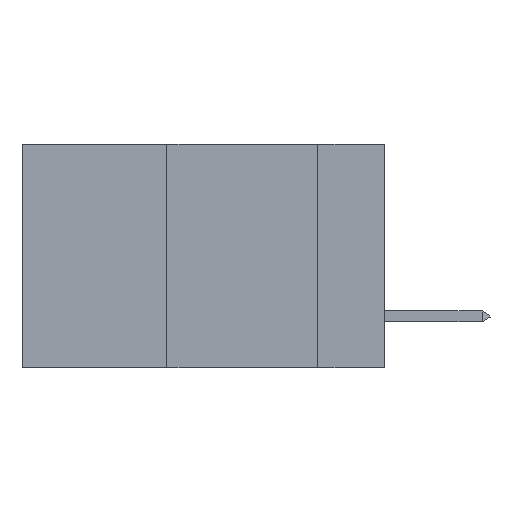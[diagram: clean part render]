
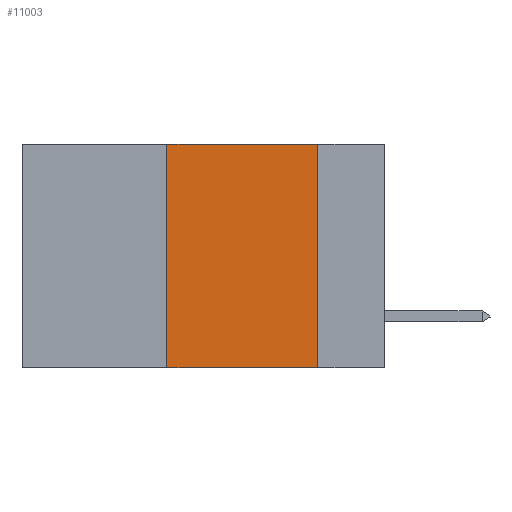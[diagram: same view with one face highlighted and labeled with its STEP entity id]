
A CAD part, left-side view. The second image highlights one B-rep face of the part: STEP entity #11003.
In plain terms, the highlighted planar face has unit normal (-1, 0, 0).
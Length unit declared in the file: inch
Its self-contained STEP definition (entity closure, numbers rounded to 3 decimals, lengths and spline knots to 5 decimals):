
#682 = VECTOR ( 'NONE', #30937, 39.37008 ) ;
#923 = PLANE ( 'NONE',  #15799 ) ;
#1161 = FACE_OUTER_BOUND ( 'NONE', #6146, .T. ) ;
#1852 = LINE ( 'NONE', #16204, #682 ) ;
#6146 = EDGE_LOOP ( 'NONE', ( #11943, #43986, #10461, #16983 ) ) ;
#6515 = LINE ( 'NONE', #18355, #30568 ) ;
#7495 = VECTOR ( 'NONE', #24805, 39.37008 ) ;
#9972 = EDGE_CURVE ( 'NONE', #40514, #22661, #1852, .T. ) ;
#10461 = ORIENTED_EDGE ( 'NONE', *, *, #11871, .F. ) ;
#11003 = ADVANCED_FACE ( 'NONE', ( #1161 ), #923, .F. ) ;
#11871 = EDGE_CURVE ( 'NONE', #40514, #37685, #32154, .T. ) ;
#11943 = ORIENTED_EDGE ( 'NONE', *, *, #27723, .F. ) ;
#12066 = DIRECTION ( 'NONE',  ( 0., 0., -1. ) ) ;
#14616 = CARTESIAN_POINT ( 'NONE',  ( 0., 0.6, 0. ) ) ;
#15799 = AXIS2_PLACEMENT_3D ( 'NONE', #30419, #22915, #12066 ) ;
#16204 = CARTESIAN_POINT ( 'NONE',  ( 0., 0.6, -0.37 ) ) ;
#16643 = CARTESIAN_POINT ( 'NONE',  ( 0., 0.36, 0. ) ) ;
#16983 = ORIENTED_EDGE ( 'NONE', *, *, #9972, .T. ) ;
#18355 = CARTESIAN_POINT ( 'NONE',  ( 0., 0.11, 0. ) ) ;
#22661 = VERTEX_POINT ( 'NONE', #30982 ) ;
#22915 = DIRECTION ( 'NONE',  ( 1., 0., 0. ) ) ;
#24805 = DIRECTION ( 'NONE',  ( 0., 0., 1. ) ) ;
#25208 = VECTOR ( 'NONE', #37719, 39.37008 ) ;
#25822 = VERTEX_POINT ( 'NONE', #32988 ) ;
#27723 = EDGE_CURVE ( 'NONE', #25822, #22661, #6515, .T. ) ;
#29859 = CARTESIAN_POINT ( 'NONE',  ( 0., 0.36, 0. ) ) ;
#30419 = CARTESIAN_POINT ( 'NONE',  ( 0., 0.6, 0. ) ) ;
#30420 = CARTESIAN_POINT ( 'NONE',  ( 0., 0.36, -0.37 ) ) ;
#30568 = VECTOR ( 'NONE', #33601, 39.37008 ) ;
#30937 = DIRECTION ( 'NONE',  ( 0., -1., 0. ) ) ;
#30982 = CARTESIAN_POINT ( 'NONE',  ( 0., 0.11, -0.37 ) ) ;
#32154 = LINE ( 'NONE', #29859, #7495 ) ;
#32988 = CARTESIAN_POINT ( 'NONE',  ( 0., 0.11, 0. ) ) ;
#33601 = DIRECTION ( 'NONE',  ( 0., 0., -1. ) ) ;
#37685 = VERTEX_POINT ( 'NONE', #16643 ) ;
#37719 = DIRECTION ( 'NONE',  ( 0., -1., 0. ) ) ;
#38711 = LINE ( 'NONE', #14616, #25208 ) ;
#40514 = VERTEX_POINT ( 'NONE', #30420 ) ;
#43986 = ORIENTED_EDGE ( 'NONE', *, *, #46624, .F. ) ;
#46624 = EDGE_CURVE ( 'NONE', #37685, #25822, #38711, .T. ) ;
